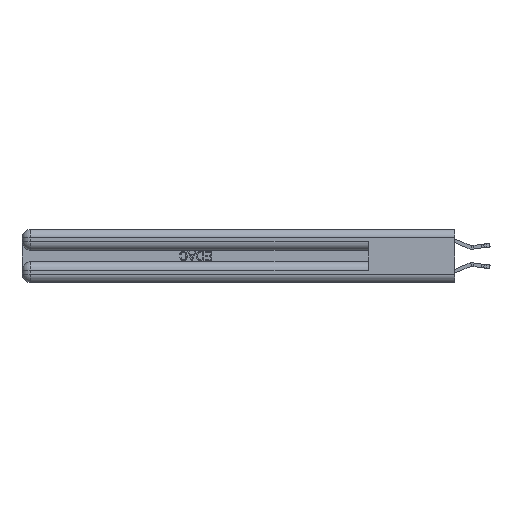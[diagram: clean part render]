
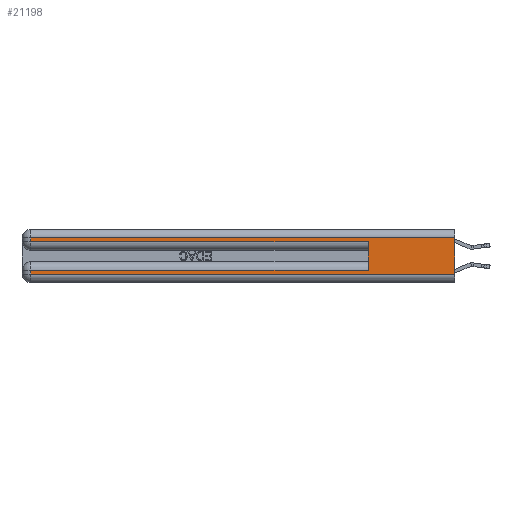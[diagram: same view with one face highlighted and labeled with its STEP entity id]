
A CAD part, left-side view. The second image highlights one B-rep face of the part: STEP entity #21198.
In plain terms, the highlighted planar face has unit normal (-1, 0, 0).
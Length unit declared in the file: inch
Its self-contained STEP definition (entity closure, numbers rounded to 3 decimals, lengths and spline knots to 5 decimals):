
#1141 = VECTOR ( 'NONE', #10735, 39.37008 ) ;
#2528 = LINE ( 'NONE', #9613, #4765 ) ;
#2733 = LINE ( 'NONE', #20135, #21675 ) ;
#4649 = LINE ( 'NONE', #4989, #18911 ) ;
#4765 = VECTOR ( 'NONE', #20106, 39.37008 ) ;
#4989 = CARTESIAN_POINT ( 'NONE',  ( 0., 0.6, 0.145 ) ) ;
#5019 = VECTOR ( 'NONE', #17504, 39.37008 ) ;
#5337 = LINE ( 'NONE', #12749, #5019 ) ;
#5965 = DIRECTION ( 'NONE',  ( 0., 0., -1. ) ) ;
#6379 = CARTESIAN_POINT ( 'NONE',  ( 0., 0.6, 0.085 ) ) ;
#6557 = EDGE_CURVE ( 'NONE', #10777, #21558, #2528, .T. ) ;
#6636 = ORIENTED_EDGE ( 'NONE', *, *, #17000, .F. ) ;
#7600 = DIRECTION ( 'NONE',  ( 0., 0., 1. ) ) ;
#7706 = EDGE_CURVE ( 'NONE', #9022, #10777, #23726, .T. ) ;
#9022 = VERTEX_POINT ( 'NONE', #6379 ) ;
#9613 = CARTESIAN_POINT ( 'NONE',  ( 0., 2.94, 0.37 ) ) ;
#10328 = LINE ( 'NONE', #15588, #23800 ) ;
#10735 = DIRECTION ( 'NONE',  ( 0., 1., 0. ) ) ;
#10777 = VERTEX_POINT ( 'NONE', #30237 ) ;
#11012 = CARTESIAN_POINT ( 'NONE',  ( 0., 0., 0.37 ) ) ;
#11307 = CARTESIAN_POINT ( 'NONE',  ( 0., 2.94, 0.06 ) ) ;
#12749 = CARTESIAN_POINT ( 'NONE',  ( 0., 0., 0.285 ) ) ;
#13036 = CARTESIAN_POINT ( 'NONE',  ( 0., 0., 0.31 ) ) ;
#14897 = VERTEX_POINT ( 'NONE', #29953 ) ;
#15588 = CARTESIAN_POINT ( 'NONE',  ( 0., 2.94, 0.37 ) ) ;
#15676 = ORIENTED_EDGE ( 'NONE', *, *, #7706, .T. ) ;
#15798 = VERTEX_POINT ( 'NONE', #30996 ) ;
#16251 = ORIENTED_EDGE ( 'NONE', *, *, #24092, .T. ) ;
#16274 = EDGE_LOOP ( 'NONE', ( #30351, #16251, #20989, #26000, #6636, #15676, #28686, #16505 ) ) ;
#16402 = CARTESIAN_POINT ( 'NONE',  ( 0., 2.94, 0.285 ) ) ;
#16433 = FACE_OUTER_BOUND ( 'NONE', #16274, .T. ) ;
#16505 = ORIENTED_EDGE ( 'NONE', *, *, #29854, .T. ) ;
#17000 = EDGE_CURVE ( 'NONE', #9022, #14897, #4649, .T. ) ;
#17504 = DIRECTION ( 'NONE',  ( 0., -1., 0. ) ) ;
#17686 = CARTESIAN_POINT ( 'NONE',  ( 0., 0., 0.31 ) ) ;
#18500 = AXIS2_PLACEMENT_3D ( 'NONE', #11012, #28365, #23784 ) ;
#18911 = VECTOR ( 'NONE', #7600, 39.37008 ) ;
#20106 = DIRECTION ( 'NONE',  ( 0., 0., -1. ) ) ;
#20135 = CARTESIAN_POINT ( 'NONE',  ( 0., 0., 0.37 ) ) ;
#20490 = DIRECTION ( 'NONE',  ( 0., 0., -1. ) ) ;
#20863 = CARTESIAN_POINT ( 'NONE',  ( 0., 0., 0.06 ) ) ;
#20989 = ORIENTED_EDGE ( 'NONE', *, *, #23230, .T. ) ;
#21198 = ADVANCED_FACE ( 'NONE', ( #16433 ), #25758, .F. ) ;
#21558 = VERTEX_POINT ( 'NONE', #11307 ) ;
#21675 = VECTOR ( 'NONE', #5965, 39.37008 ) ;
#22365 = EDGE_CURVE ( 'NONE', #25035, #31161, #2733, .T. ) ;
#23230 = EDGE_CURVE ( 'NONE', #15798, #24634, #10328, .T. ) ;
#23330 = LINE ( 'NONE', #20863, #27977 ) ;
#23396 = DIRECTION ( 'NONE',  ( 0., 1., 0. ) ) ;
#23726 = LINE ( 'NONE', #28297, #30426 ) ;
#23784 = DIRECTION ( 'NONE',  ( 0., 0., -1. ) ) ;
#23800 = VECTOR ( 'NONE', #20490, 39.37008 ) ;
#24092 = EDGE_CURVE ( 'NONE', #25035, #15798, #30360, .T. ) ;
#24634 = VERTEX_POINT ( 'NONE', #16402 ) ;
#25035 = VERTEX_POINT ( 'NONE', #17686 ) ;
#25758 = PLANE ( 'NONE',  #18500 ) ;
#25941 = DIRECTION ( 'NONE',  ( 0., -1., 0. ) ) ;
#26000 = ORIENTED_EDGE ( 'NONE', *, *, #29193, .T. ) ;
#27977 = VECTOR ( 'NONE', #25941, 39.37008 ) ;
#28297 = CARTESIAN_POINT ( 'NONE',  ( 0., 0., 0.085 ) ) ;
#28365 = DIRECTION ( 'NONE',  ( 1., 0., 0. ) ) ;
#28686 = ORIENTED_EDGE ( 'NONE', *, *, #6557, .T. ) ;
#29193 = EDGE_CURVE ( 'NONE', #24634, #14897, #5337, .T. ) ;
#29598 = CARTESIAN_POINT ( 'NONE',  ( 0., 0., 0.06 ) ) ;
#29854 = EDGE_CURVE ( 'NONE', #21558, #31161, #23330, .T. ) ;
#29953 = CARTESIAN_POINT ( 'NONE',  ( 0., 0.6, 0.285 ) ) ;
#30237 = CARTESIAN_POINT ( 'NONE',  ( 0., 2.94, 0.085 ) ) ;
#30351 = ORIENTED_EDGE ( 'NONE', *, *, #22365, .F. ) ;
#30360 = LINE ( 'NONE', #13036, #1141 ) ;
#30426 = VECTOR ( 'NONE', #23396, 39.37008 ) ;
#30996 = CARTESIAN_POINT ( 'NONE',  ( 0., 2.94, 0.31 ) ) ;
#31161 = VERTEX_POINT ( 'NONE', #29598 ) ;
